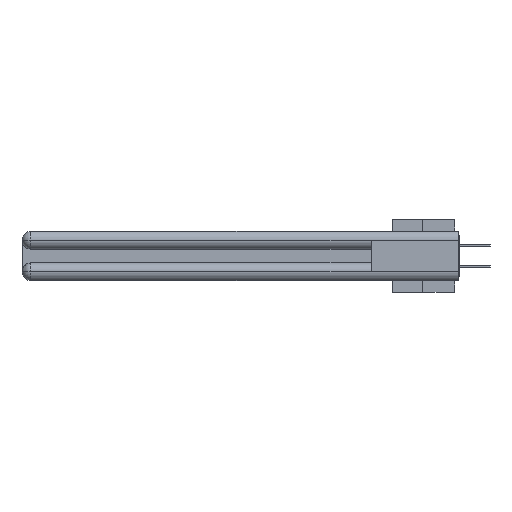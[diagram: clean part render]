
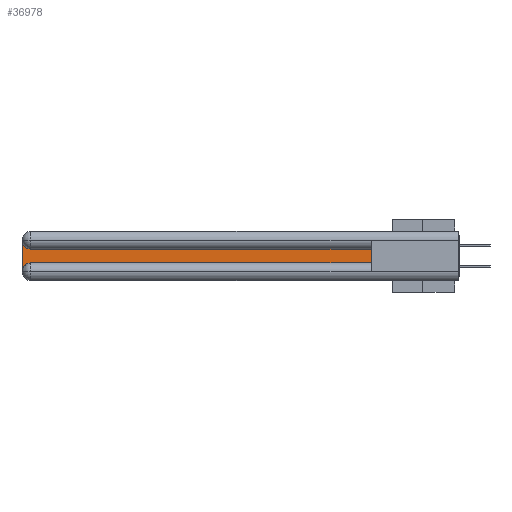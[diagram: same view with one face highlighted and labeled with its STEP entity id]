
A CAD part, left-side view. The second image highlights one B-rep face of the part: STEP entity #36978.
In plain terms, the highlighted planar face has unit normal (-1, 0, 0).
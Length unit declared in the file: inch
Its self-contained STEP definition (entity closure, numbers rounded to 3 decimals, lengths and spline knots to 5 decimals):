
#78 = EDGE_CURVE ( 'NONE', #6329, #6741, #18786, .T. ) ;
#240 = CARTESIAN_POINT ( 'NONE',  ( 0.075, 0.6, -0.2175 ) ) ;
#2519 = CARTESIAN_POINT ( 'NONE',  ( 0.075, 2.94, -0.0625 ) ) ;
#2606 = FACE_OUTER_BOUND ( 'NONE', #35389, .T. ) ;
#4251 = EDGE_CURVE ( 'NONE', #28820, #6329, #21212, .T. ) ;
#4797 = CARTESIAN_POINT ( 'NONE',  ( 0.075, 2.94, -0.2175 ) ) ;
#4814 = DIRECTION ( 'NONE',  ( 0., 0., 1. ) ) ;
#5688 = CIRCLE ( 'NONE', #22578, 0.06 ) ;
#6102 = VECTOR ( 'NONE', #25914, 39.37008 ) ;
#6329 = VERTEX_POINT ( 'NONE', #18261 ) ;
#6517 = VERTEX_POINT ( 'NONE', #4797 ) ;
#6650 = DIRECTION ( 'NONE',  ( 1., 0., 0. ) ) ;
#6675 = ORIENTED_EDGE ( 'NONE', *, *, #17555, .T. ) ;
#6741 = VERTEX_POINT ( 'NONE', #18964 ) ;
#6921 = LINE ( 'NONE', #30265, #33960 ) ;
#9222 = VECTOR ( 'NONE', #4814, 39.37008 ) ;
#9809 = DIRECTION ( 'NONE',  ( 0., 0., -1. ) ) ;
#12802 = DIRECTION ( 'NONE',  ( 1., 0., 0. ) ) ;
#14591 = EDGE_CURVE ( 'NONE', #6741, #22549, #36805, .T. ) ;
#15475 = AXIS2_PLACEMENT_3D ( 'NONE', #32765, #6650, #9809 ) ;
#17344 = DIRECTION ( 'NONE',  ( 1., 0., 0. ) ) ;
#17555 = EDGE_CURVE ( 'NONE', #6517, #28942, #6921, .T. ) ;
#18036 = VECTOR ( 'NONE', #36932, 39.37008 ) ;
#18261 = CARTESIAN_POINT ( 'NONE',  ( 0.075, 2.94, -0.1225 ) ) ;
#18786 = CIRCLE ( 'NONE', #21940, 0.06 ) ;
#18826 = CARTESIAN_POINT ( 'NONE',  ( 0.075, 2.94, -0.2775 ) ) ;
#18964 = CARTESIAN_POINT ( 'NONE',  ( 0.075, 3., -0.0625 ) ) ;
#21212 = LINE ( 'NONE', #28716, #18036 ) ;
#21923 = ORIENTED_EDGE ( 'NONE', *, *, #78, .T. ) ;
#21940 = AXIS2_PLACEMENT_3D ( 'NONE', #2519, #17344, #28782 ) ;
#22549 = VERTEX_POINT ( 'NONE', #32617 ) ;
#22578 = AXIS2_PLACEMENT_3D ( 'NONE', #18826, #12802, #27499 ) ;
#24855 = ORIENTED_EDGE ( 'NONE', *, *, #33394, .T. ) ;
#25914 = DIRECTION ( 'NONE',  ( 0., 0., -1. ) ) ;
#26941 = ORIENTED_EDGE ( 'NONE', *, *, #4251, .T. ) ;
#27478 = DIRECTION ( 'NONE',  ( 0., -1., 0. ) ) ;
#27499 = DIRECTION ( 'NONE',  ( 0., 0., -1. ) ) ;
#28234 = ORIENTED_EDGE ( 'NONE', *, *, #31433, .T. ) ;
#28716 = CARTESIAN_POINT ( 'NONE',  ( 0.075, 0.6, -0.1225 ) ) ;
#28782 = DIRECTION ( 'NONE',  ( 0., 0., -1. ) ) ;
#28820 = VERTEX_POINT ( 'NONE', #31826 ) ;
#28942 = VERTEX_POINT ( 'NONE', #240 ) ;
#29973 = LINE ( 'NONE', #30471, #9222 ) ;
#30265 = CARTESIAN_POINT ( 'NONE',  ( 0.075, 0.6, -0.2175 ) ) ;
#30471 = CARTESIAN_POINT ( 'NONE',  ( 0.075, 0.6, -0.2175 ) ) ;
#31433 = EDGE_CURVE ( 'NONE', #22549, #6517, #5688, .T. ) ;
#31826 = CARTESIAN_POINT ( 'NONE',  ( 0.075, 0.6, -0.1225 ) ) ;
#32520 = PLANE ( 'NONE',  #15475 ) ;
#32617 = CARTESIAN_POINT ( 'NONE',  ( 0.075, 3., -0.2775 ) ) ;
#32765 = CARTESIAN_POINT ( 'NONE',  ( 0.075, 3., -0.1225 ) ) ;
#33394 = EDGE_CURVE ( 'NONE', #28942, #28820, #29973, .T. ) ;
#33960 = VECTOR ( 'NONE', #27478, 39.37008 ) ;
#34269 = ORIENTED_EDGE ( 'NONE', *, *, #14591, .T. ) ;
#35389 = EDGE_LOOP ( 'NONE', ( #26941, #21923, #34269, #28234, #6675, #24855 ) ) ;
#36805 = LINE ( 'NONE', #37375, #6102 ) ;
#36932 = DIRECTION ( 'NONE',  ( 0., 1., 0. ) ) ;
#36978 = ADVANCED_FACE ( 'NONE', ( #2606 ), #32520, .F. ) ;
#37375 = CARTESIAN_POINT ( 'NONE',  ( 0.075, 3., -0.2175 ) ) ;
